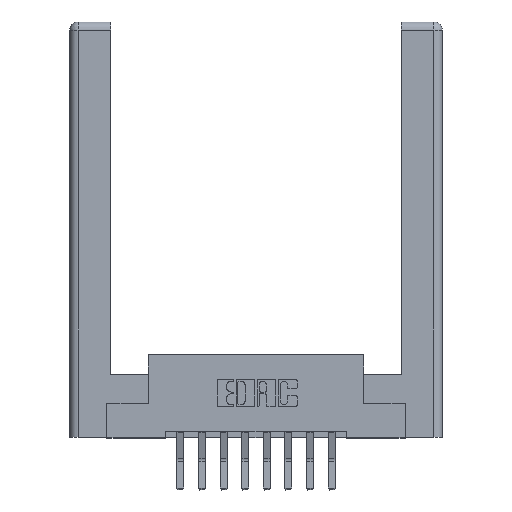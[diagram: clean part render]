
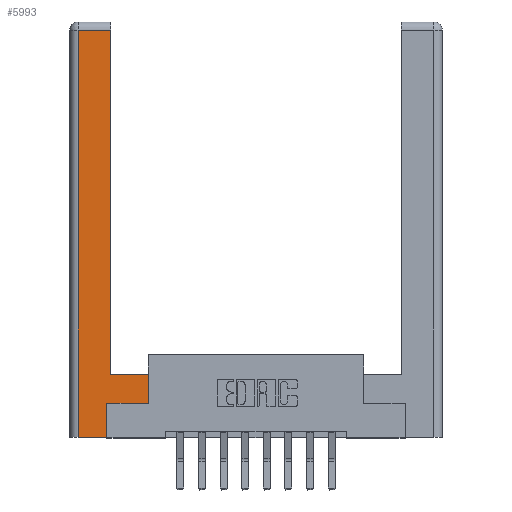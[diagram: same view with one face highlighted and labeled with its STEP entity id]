
A CAD part, top view. The second image highlights one B-rep face of the part: STEP entity #5993.
In plain terms, the highlighted planar face has unit normal (0, 0, 1).
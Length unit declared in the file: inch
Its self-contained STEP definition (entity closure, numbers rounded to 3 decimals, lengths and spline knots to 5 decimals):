
#195 = DIRECTION ( 'NONE',  ( 1., 0., 0. ) ) ;
#555 = VECTOR ( 'NONE', #6714, 39.37008 ) ;
#922 = CARTESIAN_POINT ( 'NONE',  ( 0.0615, 0., 0. ) ) ;
#1086 = CARTESIAN_POINT ( 'NONE',  ( 0.0615, 2.94, 0. ) ) ;
#1175 = VERTEX_POINT ( 'NONE', #922 ) ;
#1612 = CARTESIAN_POINT ( 'NONE',  ( 0.265, 0.245, 0. ) ) ;
#1826 = EDGE_CURVE ( 'NONE', #9776, #1175, #6236, .T. ) ;
#2225 = VECTOR ( 'NONE', #8319, 39.37008 ) ;
#2302 = VECTOR ( 'NONE', #3736, 39.37008 ) ;
#2557 = ORIENTED_EDGE ( 'NONE', *, *, #7442, .T. ) ;
#2913 = AXIS2_PLACEMENT_3D ( 'NONE', #13188, #13000, #12118 ) ;
#3197 = ORIENTED_EDGE ( 'NONE', *, *, #5871, .T. ) ;
#3685 = CARTESIAN_POINT ( 'NONE',  ( 0.295, 2.94, 0. ) ) ;
#3736 = DIRECTION ( 'NONE',  ( 0., 1., 0. ) ) ;
#3749 = CARTESIAN_POINT ( 'NONE',  ( 0.0615, 0., 0. ) ) ;
#3977 = ORIENTED_EDGE ( 'NONE', *, *, #1826, .T. ) ;
#4210 = LINE ( 'NONE', #1086, #2225 ) ;
#4239 = LINE ( 'NONE', #4372, #5044 ) ;
#4372 = CARTESIAN_POINT ( 'NONE',  ( 0.565, 0.245, 0. ) ) ;
#4457 = CARTESIAN_POINT ( 'NONE',  ( 0.565, 0.245, 0. ) ) ;
#4593 = ORIENTED_EDGE ( 'NONE', *, *, #5176, .T. ) ;
#4794 = DIRECTION ( 'NONE',  ( -1., 0., 0. ) ) ;
#5044 = VECTOR ( 'NONE', #195, 39.37008 ) ;
#5067 = LINE ( 'NONE', #10918, #9038 ) ;
#5176 = EDGE_CURVE ( 'NONE', #10618, #12403, #5252, .T. ) ;
#5219 = VERTEX_POINT ( 'NONE', #1612 ) ;
#5252 = LINE ( 'NONE', #11807, #2302 ) ;
#5631 = LINE ( 'NONE', #10939, #555 ) ;
#5871 = EDGE_CURVE ( 'NONE', #12403, #11360, #5067, .T. ) ;
#5993 = ADVANCED_FACE ( 'NONE', ( #10160 ), #10051, .F. ) ;
#6236 = LINE ( 'NONE', #3749, #6720 ) ;
#6279 = ORIENTED_EDGE ( 'NONE', *, *, #9385, .T. ) ;
#6714 = DIRECTION ( 'NONE',  ( 0., 1., 0. ) ) ;
#6720 = VECTOR ( 'NONE', #7882, 39.37008 ) ;
#6844 = VERTEX_POINT ( 'NONE', #9195 ) ;
#7029 = CARTESIAN_POINT ( 'NONE',  ( 0.565, 0.45, 0. ) ) ;
#7238 = ORIENTED_EDGE ( 'NONE', *, *, #10649, .T. ) ;
#7442 = EDGE_CURVE ( 'NONE', #1175, #6844, #8820, .T. ) ;
#7882 = DIRECTION ( 'NONE',  ( 0., -1., 0. ) ) ;
#8114 = DIRECTION ( 'NONE',  ( 1., 0., 0. ) ) ;
#8161 = EDGE_LOOP ( 'NONE', ( #10046, #10371, #3977, #2557, #6279, #7238, #4593, #3197 ) ) ;
#8319 = DIRECTION ( 'NONE',  ( -1., 0., 0. ) ) ;
#8500 = VECTOR ( 'NONE', #12703, 39.37008 ) ;
#8559 = CARTESIAN_POINT ( 'NONE',  ( 0.0615, 2.94, 0. ) ) ;
#8715 = EDGE_CURVE ( 'NONE', #11360, #11934, #9948, .T. ) ;
#8820 = LINE ( 'NONE', #10101, #13328 ) ;
#9038 = VECTOR ( 'NONE', #4794, 39.37008 ) ;
#9195 = CARTESIAN_POINT ( 'NONE',  ( 0.265, 0., 0. ) ) ;
#9385 = EDGE_CURVE ( 'NONE', #6844, #5219, #5631, .T. ) ;
#9776 = VERTEX_POINT ( 'NONE', #8559 ) ;
#9948 = LINE ( 'NONE', #10645, #8500 ) ;
#10046 = ORIENTED_EDGE ( 'NONE', *, *, #8715, .T. ) ;
#10051 = PLANE ( 'NONE',  #2913 ) ;
#10101 = CARTESIAN_POINT ( 'NONE',  ( 0.265, 0., 0. ) ) ;
#10160 = FACE_OUTER_BOUND ( 'NONE', #8161, .T. ) ;
#10371 = ORIENTED_EDGE ( 'NONE', *, *, #11683, .T. ) ;
#10582 = CARTESIAN_POINT ( 'NONE',  ( 0.295, 0.45, 0. ) ) ;
#10618 = VERTEX_POINT ( 'NONE', #4457 ) ;
#10645 = CARTESIAN_POINT ( 'NONE',  ( 0.295, 3., 0. ) ) ;
#10649 = EDGE_CURVE ( 'NONE', #5219, #10618, #4239, .T. ) ;
#10918 = CARTESIAN_POINT ( 'NONE',  ( 0.295, 0.45, 0. ) ) ;
#10939 = CARTESIAN_POINT ( 'NONE',  ( 0.265, 0.245, 0. ) ) ;
#11360 = VERTEX_POINT ( 'NONE', #10582 ) ;
#11683 = EDGE_CURVE ( 'NONE', #11934, #9776, #4210, .T. ) ;
#11807 = CARTESIAN_POINT ( 'NONE',  ( 0.565, 0.45, 0. ) ) ;
#11934 = VERTEX_POINT ( 'NONE', #3685 ) ;
#12118 = DIRECTION ( 'NONE',  ( -1., 0., 0. ) ) ;
#12403 = VERTEX_POINT ( 'NONE', #7029 ) ;
#12703 = DIRECTION ( 'NONE',  ( 0., 1., 0. ) ) ;
#13000 = DIRECTION ( 'NONE',  ( 0., 0., -1. ) ) ;
#13188 = CARTESIAN_POINT ( 'NONE',  ( 0., 0., 0. ) ) ;
#13328 = VECTOR ( 'NONE', #8114, 39.37008 ) ;
